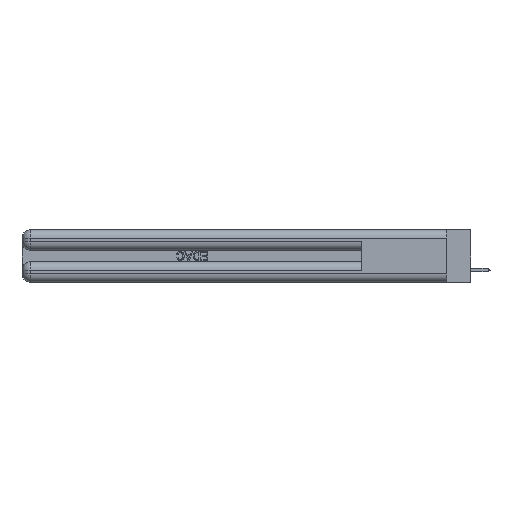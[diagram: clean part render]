
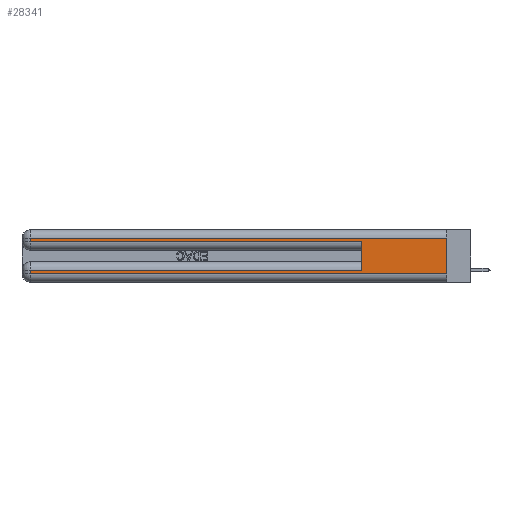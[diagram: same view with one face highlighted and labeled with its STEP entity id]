
A CAD part, left-side view. The second image highlights one B-rep face of the part: STEP entity #28341.
In plain terms, the highlighted planar face has unit normal (-1, 0, 0).
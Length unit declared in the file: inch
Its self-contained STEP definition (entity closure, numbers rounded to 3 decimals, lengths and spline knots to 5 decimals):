
#871 = VECTOR ( 'NONE', #40443, 39.37008 ) ;
#1227 = VECTOR ( 'NONE', #22927, 39.37008 ) ;
#1920 = VECTOR ( 'NONE', #17309, 39.37008 ) ;
#1952 = EDGE_CURVE ( 'NONE', #14652, #7301, #13417, .T. ) ;
#2326 = DIRECTION ( 'NONE',  ( 0., 0., -1. ) ) ;
#3001 = CARTESIAN_POINT ( 'NONE',  ( 0., 0., 0.06 ) ) ;
#3130 = EDGE_CURVE ( 'NONE', #18593, #14248, #37546, .T. ) ;
#3315 = DIRECTION ( 'NONE',  ( 0., 1., 0. ) ) ;
#4800 = CARTESIAN_POINT ( 'NONE',  ( 0., 0., 0.37 ) ) ;
#6227 = ORIENTED_EDGE ( 'NONE', *, *, #29779, .T. ) ;
#6335 = CARTESIAN_POINT ( 'NONE',  ( 0., 0., 0.31 ) ) ;
#7007 = VECTOR ( 'NONE', #2326, 39.37008 ) ;
#7301 = VERTEX_POINT ( 'NONE', #8156 ) ;
#7743 = LINE ( 'NONE', #30040, #41589 ) ;
#8156 = CARTESIAN_POINT ( 'NONE',  ( 0., 2.94, 0.06 ) ) ;
#8173 = PLANE ( 'NONE',  #16685 ) ;
#8878 = ORIENTED_EDGE ( 'NONE', *, *, #3130, .T. ) ;
#10185 = LINE ( 'NONE', #3001, #1227 ) ;
#12341 = VECTOR ( 'NONE', #33589, 39.37008 ) ;
#12543 = ORIENTED_EDGE ( 'NONE', *, *, #1952, .T. ) ;
#13417 = LINE ( 'NONE', #22083, #7007 ) ;
#13701 = VERTEX_POINT ( 'NONE', #28006 ) ;
#14248 = VERTEX_POINT ( 'NONE', #39930 ) ;
#14652 = VERTEX_POINT ( 'NONE', #42544 ) ;
#15875 = ORIENTED_EDGE ( 'NONE', *, *, #41094, .F. ) ;
#16685 = AXIS2_PLACEMENT_3D ( 'NONE', #4800, #25191, #18124 ) ;
#17309 = DIRECTION ( 'NONE',  ( 0., 0., -1. ) ) ;
#17657 = LINE ( 'NONE', #33164, #12341 ) ;
#18124 = DIRECTION ( 'NONE',  ( 0., 0., -1. ) ) ;
#18593 = VERTEX_POINT ( 'NONE', #37939 ) ;
#18826 = ORIENTED_EDGE ( 'NONE', *, *, #28614, .T. ) ;
#18895 = FACE_OUTER_BOUND ( 'NONE', #28574, .T. ) ;
#20521 = ORIENTED_EDGE ( 'NONE', *, *, #21639, .T. ) ;
#21639 = EDGE_CURVE ( 'NONE', #14248, #13701, #29942, .T. ) ;
#22083 = CARTESIAN_POINT ( 'NONE',  ( 0., 2.94, 0.37 ) ) ;
#22927 = DIRECTION ( 'NONE',  ( 0., -1., 0. ) ) ;
#23732 = EDGE_CURVE ( 'NONE', #7301, #37567, #10185, .T. ) ;
#23786 = VERTEX_POINT ( 'NONE', #40188 ) ;
#24011 = LINE ( 'NONE', #35828, #37713 ) ;
#25191 = DIRECTION ( 'NONE',  ( 1., 0., 0. ) ) ;
#25955 = VERTEX_POINT ( 'NONE', #27776 ) ;
#27552 = VECTOR ( 'NONE', #40149, 39.37008 ) ;
#27649 = ORIENTED_EDGE ( 'NONE', *, *, #23732, .T. ) ;
#27776 = CARTESIAN_POINT ( 'NONE',  ( 0., 0.6, 0.285 ) ) ;
#28006 = CARTESIAN_POINT ( 'NONE',  ( 0., 2.94, 0.285 ) ) ;
#28341 = ADVANCED_FACE ( 'NONE', ( #18895 ), #8173, .F. ) ;
#28574 = EDGE_LOOP ( 'NONE', ( #39597, #8878, #20521, #6227, #15875, #18826, #12543, #27649 ) ) ;
#28614 = EDGE_CURVE ( 'NONE', #23786, #14652, #7743, .T. ) ;
#29779 = EDGE_CURVE ( 'NONE', #13701, #25955, #24011, .T. ) ;
#29942 = LINE ( 'NONE', #37488, #1920 ) ;
#30040 = CARTESIAN_POINT ( 'NONE',  ( 0., 0., 0.085 ) ) ;
#33164 = CARTESIAN_POINT ( 'NONE',  ( 0., 0., 0.37 ) ) ;
#33589 = DIRECTION ( 'NONE',  ( 0., 0., -1. ) ) ;
#34609 = LINE ( 'NONE', #40888, #871 ) ;
#35828 = CARTESIAN_POINT ( 'NONE',  ( 0., 0., 0.285 ) ) ;
#37488 = CARTESIAN_POINT ( 'NONE',  ( 0., 2.94, 0.37 ) ) ;
#37546 = LINE ( 'NONE', #6335, #27552 ) ;
#37567 = VERTEX_POINT ( 'NONE', #39781 ) ;
#37713 = VECTOR ( 'NONE', #40161, 39.37008 ) ;
#37939 = CARTESIAN_POINT ( 'NONE',  ( 0., 0., 0.31 ) ) ;
#39597 = ORIENTED_EDGE ( 'NONE', *, *, #42396, .F. ) ;
#39781 = CARTESIAN_POINT ( 'NONE',  ( 0., 0., 0.06 ) ) ;
#39930 = CARTESIAN_POINT ( 'NONE',  ( 0., 2.94, 0.31 ) ) ;
#40149 = DIRECTION ( 'NONE',  ( 0., 1., 0. ) ) ;
#40161 = DIRECTION ( 'NONE',  ( 0., -1., 0. ) ) ;
#40188 = CARTESIAN_POINT ( 'NONE',  ( 0., 0.6, 0.085 ) ) ;
#40443 = DIRECTION ( 'NONE',  ( 0., 0., 1. ) ) ;
#40888 = CARTESIAN_POINT ( 'NONE',  ( 0., 0.6, 0.145 ) ) ;
#41094 = EDGE_CURVE ( 'NONE', #23786, #25955, #34609, .T. ) ;
#41589 = VECTOR ( 'NONE', #3315, 39.37008 ) ;
#42396 = EDGE_CURVE ( 'NONE', #18593, #37567, #17657, .T. ) ;
#42544 = CARTESIAN_POINT ( 'NONE',  ( 0., 2.94, 0.085 ) ) ;
